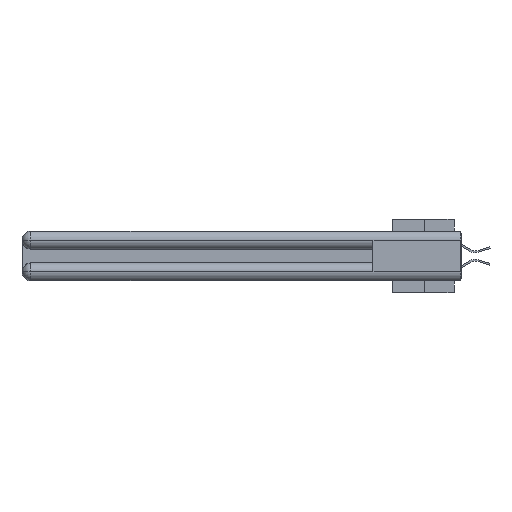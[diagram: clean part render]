
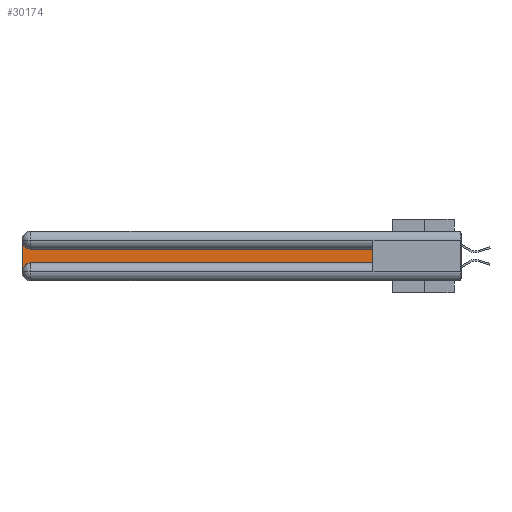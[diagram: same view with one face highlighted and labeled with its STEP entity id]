
A CAD part, left-side view. The second image highlights one B-rep face of the part: STEP entity #30174.
In plain terms, the highlighted planar face has unit normal (-1, 0, 0).
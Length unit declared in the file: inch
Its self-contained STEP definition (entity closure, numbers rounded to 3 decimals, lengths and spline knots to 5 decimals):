
#89 = EDGE_CURVE ( 'NONE', #15545, #2058, #18899, .T. ) ;
#598 = EDGE_CURVE ( 'NONE', #32584, #14080, #30719, .T. ) ;
#1521 = CARTESIAN_POINT ( 'NONE',  ( 0.075, 3., -0.0625 ) ) ;
#2058 = VERTEX_POINT ( 'NONE', #28470 ) ;
#2133 = LINE ( 'NONE', #3736, #35669 ) ;
#2397 = EDGE_CURVE ( 'NONE', #31126, #15545, #20709, .T. ) ;
#3736 = CARTESIAN_POINT ( 'NONE',  ( 0.075, 3., -0.2175 ) ) ;
#4801 = ORIENTED_EDGE ( 'NONE', *, *, #27499, .T. ) ;
#5093 = VECTOR ( 'NONE', #39209, 39.37008 ) ;
#6832 = ORIENTED_EDGE ( 'NONE', *, *, #12664, .T. ) ;
#6909 = DIRECTION ( 'NONE',  ( 0., 0., -1. ) ) ;
#7777 = EDGE_LOOP ( 'NONE', ( #4801, #17652, #25601, #17846, #30783, #6832 ) ) ;
#11155 = CARTESIAN_POINT ( 'NONE',  ( 0.075, 3., -0.1225 ) ) ;
#11178 = DIRECTION ( 'NONE',  ( 0., 0., -1. ) ) ;
#11458 = DIRECTION ( 'NONE',  ( 1., 0., 0. ) ) ;
#11760 = CARTESIAN_POINT ( 'NONE',  ( 0.075, 0.6, -0.2175 ) ) ;
#12664 = EDGE_CURVE ( 'NONE', #2058, #35759, #26023, .T. ) ;
#12872 = CARTESIAN_POINT ( 'NONE',  ( 0.075, 2.94, -0.1225 ) ) ;
#13009 = CARTESIAN_POINT ( 'NONE',  ( 0.075, 2.94, -0.0625 ) ) ;
#14080 = VERTEX_POINT ( 'NONE', #1521 ) ;
#14333 = DIRECTION ( 'NONE',  ( 0., 0., -1. ) ) ;
#15545 = VERTEX_POINT ( 'NONE', #34355 ) ;
#17383 = AXIS2_PLACEMENT_3D ( 'NONE', #13009, #35084, #22542 ) ;
#17652 = ORIENTED_EDGE ( 'NONE', *, *, #598, .T. ) ;
#17694 = VECTOR ( 'NONE', #30542, 39.37008 ) ;
#17846 = ORIENTED_EDGE ( 'NONE', *, *, #2397, .T. ) ;
#18899 = LINE ( 'NONE', #38126, #5093 ) ;
#20687 = PLANE ( 'NONE',  #27702 ) ;
#20709 = CIRCLE ( 'NONE', #25869, 0.06 ) ;
#21019 = CARTESIAN_POINT ( 'NONE',  ( 0.075, 2.94, -0.2775 ) ) ;
#21820 = CARTESIAN_POINT ( 'NONE',  ( 0.075, 0.6, -0.1225 ) ) ;
#22266 = CARTESIAN_POINT ( 'NONE',  ( 0.075, 3., -0.2775 ) ) ;
#22372 = VECTOR ( 'NONE', #37816, 39.37008 ) ;
#22542 = DIRECTION ( 'NONE',  ( 0., 0., -1. ) ) ;
#25601 = ORIENTED_EDGE ( 'NONE', *, *, #32696, .T. ) ;
#25869 = AXIS2_PLACEMENT_3D ( 'NONE', #21019, #11458, #11178 ) ;
#26023 = LINE ( 'NONE', #11760, #17694 ) ;
#27499 = EDGE_CURVE ( 'NONE', #35759, #32584, #35172, .T. ) ;
#27702 = AXIS2_PLACEMENT_3D ( 'NONE', #11155, #33233, #14333 ) ;
#28470 = CARTESIAN_POINT ( 'NONE',  ( 0.075, 0.6, -0.2175 ) ) ;
#30174 = ADVANCED_FACE ( 'NONE', ( #39825 ), #20687, .F. ) ;
#30542 = DIRECTION ( 'NONE',  ( 0., 0., 1. ) ) ;
#30719 = CIRCLE ( 'NONE', #17383, 0.06 ) ;
#30783 = ORIENTED_EDGE ( 'NONE', *, *, #89, .T. ) ;
#31126 = VERTEX_POINT ( 'NONE', #22266 ) ;
#31280 = CARTESIAN_POINT ( 'NONE',  ( 0.075, 0.6, -0.1225 ) ) ;
#32584 = VERTEX_POINT ( 'NONE', #12872 ) ;
#32696 = EDGE_CURVE ( 'NONE', #14080, #31126, #2133, .T. ) ;
#33233 = DIRECTION ( 'NONE',  ( 1., 0., 0. ) ) ;
#34355 = CARTESIAN_POINT ( 'NONE',  ( 0.075, 2.94, -0.2175 ) ) ;
#35084 = DIRECTION ( 'NONE',  ( 1., 0., 0. ) ) ;
#35172 = LINE ( 'NONE', #21820, #22372 ) ;
#35669 = VECTOR ( 'NONE', #6909, 39.37008 ) ;
#35759 = VERTEX_POINT ( 'NONE', #31280 ) ;
#37816 = DIRECTION ( 'NONE',  ( 0., 1., 0. ) ) ;
#38126 = CARTESIAN_POINT ( 'NONE',  ( 0.075, 0.6, -0.2175 ) ) ;
#39209 = DIRECTION ( 'NONE',  ( 0., -1., 0. ) ) ;
#39825 = FACE_OUTER_BOUND ( 'NONE', #7777, .T. ) ;
